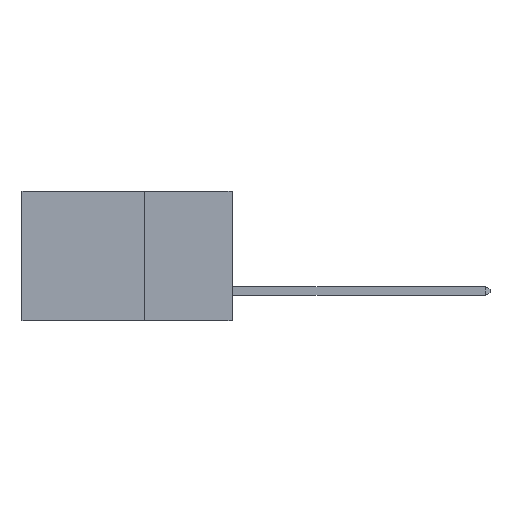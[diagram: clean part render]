
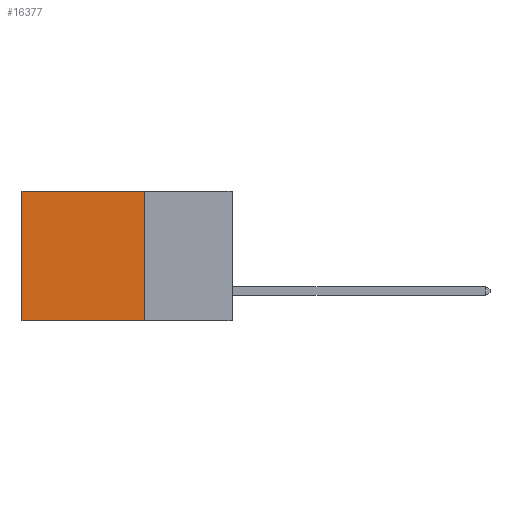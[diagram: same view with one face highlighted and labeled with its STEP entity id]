
A CAD part, left-side view. The second image highlights one B-rep face of the part: STEP entity #16377.
In plain terms, the highlighted planar face has unit normal (-1, 0, 0).
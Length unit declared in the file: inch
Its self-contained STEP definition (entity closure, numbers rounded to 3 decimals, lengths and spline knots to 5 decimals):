
#2674 = CARTESIAN_POINT ( 'NONE',  ( 0.2875, 0.25, -0.37 ) ) ;
#3208 = CARTESIAN_POINT ( 'NONE',  ( 0.2875, 0.25, 0. ) ) ;
#5273 = VECTOR ( 'NONE', #12608, 39.37008 ) ;
#5478 = DIRECTION ( 'NONE',  ( 0., 0., -1. ) ) ;
#5508 = CARTESIAN_POINT ( 'NONE',  ( 0.2875, 0.6, 0. ) ) ;
#7346 = EDGE_CURVE ( 'NONE', #13382, #26627, #14300, .T. ) ;
#7678 = ORIENTED_EDGE ( 'NONE', *, *, #26899, .F. ) ;
#7752 = DIRECTION ( 'NONE',  ( 0., 0., -1. ) ) ;
#8302 = CARTESIAN_POINT ( 'NONE',  ( 0.2875, 0.6, 0. ) ) ;
#8373 = LINE ( 'NONE', #14762, #5273 ) ;
#8679 = FACE_OUTER_BOUND ( 'NONE', #11495, .T. ) ;
#9281 = ORIENTED_EDGE ( 'NONE', *, *, #13963, .T. ) ;
#10365 = DIRECTION ( 'NONE',  ( 0., 1., 0. ) ) ;
#10875 = VECTOR ( 'NONE', #7752, 39.37008 ) ;
#11126 = VECTOR ( 'NONE', #10365, 39.37008 ) ;
#11495 = EDGE_LOOP ( 'NONE', ( #9281, #7678, #14172, #21008 ) ) ;
#12608 = DIRECTION ( 'NONE',  ( 0., 1., 0. ) ) ;
#13382 = VERTEX_POINT ( 'NONE', #13484 ) ;
#13484 = CARTESIAN_POINT ( 'NONE',  ( 0.2875, 0.25, 0. ) ) ;
#13830 = DIRECTION ( 'NONE',  ( 0., 0., -1. ) ) ;
#13963 = EDGE_CURVE ( 'NONE', #14155, #24893, #23260, .T. ) ;
#14155 = VERTEX_POINT ( 'NONE', #8302 ) ;
#14172 = ORIENTED_EDGE ( 'NONE', *, *, #7346, .F. ) ;
#14300 = LINE ( 'NONE', #24772, #25267 ) ;
#14762 = CARTESIAN_POINT ( 'NONE',  ( 0.2875, 0.25, -0.37 ) ) ;
#16377 = ADVANCED_FACE ( 'NONE', ( #8679 ), #22944, .F. ) ;
#16892 = CARTESIAN_POINT ( 'NONE',  ( 0.2875, 0.25, 0. ) ) ;
#18597 = DIRECTION ( 'NONE',  ( 1., 0., 0. ) ) ;
#20119 = EDGE_CURVE ( 'NONE', #13382, #14155, #22824, .T. ) ;
#21008 = ORIENTED_EDGE ( 'NONE', *, *, #20119, .T. ) ;
#22709 = AXIS2_PLACEMENT_3D ( 'NONE', #3208, #18597, #5478 ) ;
#22824 = LINE ( 'NONE', #16892, #11126 ) ;
#22944 = PLANE ( 'NONE',  #22709 ) ;
#23260 = LINE ( 'NONE', #5508, #10875 ) ;
#24772 = CARTESIAN_POINT ( 'NONE',  ( 0.2875, 0.25, 0. ) ) ;
#24893 = VERTEX_POINT ( 'NONE', #25820 ) ;
#25267 = VECTOR ( 'NONE', #13830, 39.37008 ) ;
#25820 = CARTESIAN_POINT ( 'NONE',  ( 0.2875, 0.6, -0.37 ) ) ;
#26627 = VERTEX_POINT ( 'NONE', #2674 ) ;
#26899 = EDGE_CURVE ( 'NONE', #26627, #24893, #8373, .T. ) ;
